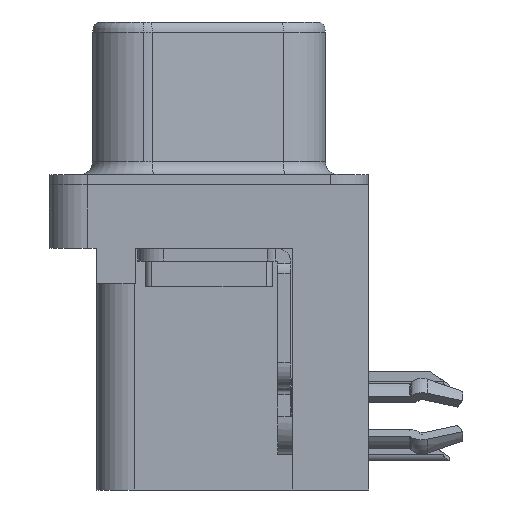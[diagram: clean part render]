
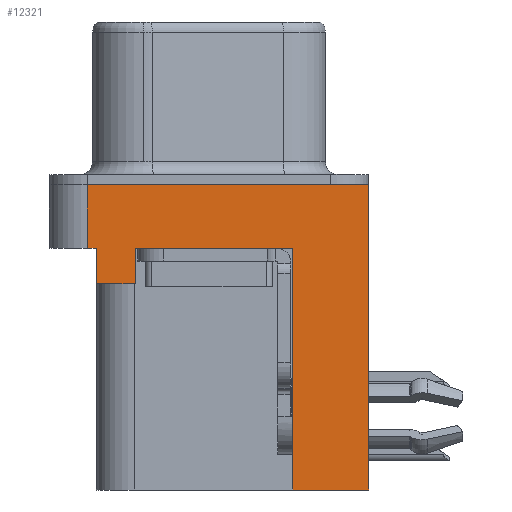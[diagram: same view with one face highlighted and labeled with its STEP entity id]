
A CAD part, left-side view. The second image highlights one B-rep face of the part: STEP entity #12321.
In plain terms, the highlighted planar face has unit normal (-1, 0, 0).
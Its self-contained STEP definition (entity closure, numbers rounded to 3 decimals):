
#18 = ORIENTED_EDGE ( 'NONE', *, *, #7341, .T. ) ;
#335 = CARTESIAN_POINT ( 'NONE',  ( -2.935, 4.775, -2.5 ) ) ;
#513 = CARTESIAN_POINT ( 'NONE',  ( -2.935, -3.295, -12. ) ) ;
#672 = VERTEX_POINT ( 'NONE', #10920 ) ;
#722 = DIRECTION ( 'NONE',  ( 0., 0., 1. ) ) ;
#1163 = CARTESIAN_POINT ( 'NONE',  ( -2.935, 2.895, -3.9 ) ) ;
#1334 = CARTESIAN_POINT ( 'NONE',  ( -2.935, -6.275, -2.5 ) ) ;
#1513 = ORIENTED_EDGE ( 'NONE', *, *, #6438, .F. ) ;
#1827 = VERTEX_POINT ( 'NONE', #1865 ) ;
#1865 = CARTESIAN_POINT ( 'NONE',  ( -2.935, 4.425, -3.9 ) ) ;
#2454 = AXIS2_PLACEMENT_3D ( 'NONE', #10579, #3220, #3462 ) ;
#2674 = LINE ( 'NONE', #13492, #13700 ) ;
#2811 = VECTOR ( 'NONE', #12744, 1000. ) ;
#2860 = LINE ( 'NONE', #6328, #15958 ) ;
#3008 = EDGE_CURVE ( 'NONE', #16433, #11795, #17096, .T. ) ;
#3125 = LINE ( 'NONE', #8642, #9172 ) ;
#3220 = DIRECTION ( 'NONE',  ( -1., 0., 0. ) ) ;
#3462 = DIRECTION ( 'NONE',  ( 0., 0., 1. ) ) ;
#3637 = CARTESIAN_POINT ( 'NONE',  ( -2.935, 2.895, -3.9 ) ) ;
#3792 = CARTESIAN_POINT ( 'NONE',  ( -2.935, 4.425, -3.9 ) ) ;
#3896 = CARTESIAN_POINT ( 'NONE',  ( -2.935, -6.275, -12. ) ) ;
#4034 = CARTESIAN_POINT ( 'NONE',  ( -2.935, -3.295, -12. ) ) ;
#4116 = LINE ( 'NONE', #3792, #15148 ) ;
#4424 = EDGE_CURVE ( 'NONE', #16189, #7552, #14632, .T. ) ;
#4591 = LINE ( 'NONE', #1334, #2811 ) ;
#5138 = VECTOR ( 'NONE', #6899, 1000. ) ;
#5188 = EDGE_CURVE ( 'NONE', #7552, #11795, #16511, .T. ) ;
#5221 = VECTOR ( 'NONE', #9967, 1000. ) ;
#5571 = VERTEX_POINT ( 'NONE', #3896 ) ;
#5678 = ORIENTED_EDGE ( 'NONE', *, *, #18589, .F. ) ;
#5716 = VERTEX_POINT ( 'NONE', #335 ) ;
#6162 = FACE_OUTER_BOUND ( 'NONE', #16030, .T. ) ;
#6328 = CARTESIAN_POINT ( 'NONE',  ( -2.935, -6.275, -2.5 ) ) ;
#6438 = EDGE_CURVE ( 'NONE', #1827, #12962, #2674, .T. ) ;
#6899 = DIRECTION ( 'NONE',  ( 0., 0., 1. ) ) ;
#7181 = CARTESIAN_POINT ( 'NONE',  ( -2.935, 4.775, -2.5 ) ) ;
#7341 = EDGE_CURVE ( 'NONE', #5716, #12962, #2860, .T. ) ;
#7552 = VERTEX_POINT ( 'NONE', #15807 ) ;
#7941 = CARTESIAN_POINT ( 'NONE',  ( -2.935, -3.295, -2.5 ) ) ;
#8073 = DIRECTION ( 'NONE',  ( 0., -1., 0. ) ) ;
#8179 = VERTEX_POINT ( 'NONE', #17858 ) ;
#8319 = VECTOR ( 'NONE', #17283, 1000. ) ;
#8461 = ORIENTED_EDGE ( 'NONE', *, *, #17868, .F. ) ;
#8642 = CARTESIAN_POINT ( 'NONE',  ( -2.935, -6.275, 0. ) ) ;
#8718 = EDGE_CURVE ( 'NONE', #5571, #672, #4591, .T. ) ;
#9172 = VECTOR ( 'NONE', #15888, 1000. ) ;
#9367 = VECTOR ( 'NONE', #18706, 1000. ) ;
#9967 = DIRECTION ( 'NONE',  ( 0., 0., 1. ) ) ;
#10202 = EDGE_CURVE ( 'NONE', #5716, #8179, #12670, .T. ) ;
#10428 = ORIENTED_EDGE ( 'NONE', *, *, #10202, .F. ) ;
#10579 = CARTESIAN_POINT ( 'NONE',  ( -2.935, -6.275, -2.5 ) ) ;
#10849 = DIRECTION ( 'NONE',  ( 0., 1., 0. ) ) ;
#10920 = CARTESIAN_POINT ( 'NONE',  ( -2.935, -6.275, 0. ) ) ;
#11165 = DIRECTION ( 'NONE',  ( 0., 1., 0. ) ) ;
#11351 = ORIENTED_EDGE ( 'NONE', *, *, #5188, .T. ) ;
#11795 = VERTEX_POINT ( 'NONE', #7941 ) ;
#12321 = ADVANCED_FACE ( 'NONE', ( #6162 ), #14818, .T. ) ;
#12621 = CARTESIAN_POINT ( 'NONE',  ( -2.935, 4.425, -2.5 ) ) ;
#12670 = LINE ( 'NONE', #7181, #5221 ) ;
#12744 = DIRECTION ( 'NONE',  ( 0., 0., 1. ) ) ;
#12962 = VERTEX_POINT ( 'NONE', #12621 ) ;
#13492 = CARTESIAN_POINT ( 'NONE',  ( -2.935, 4.425, -3.9 ) ) ;
#13700 = VECTOR ( 'NONE', #722, 1000. ) ;
#13840 = ORIENTED_EDGE ( 'NONE', *, *, #3008, .F. ) ;
#13915 = ORIENTED_EDGE ( 'NONE', *, *, #15385, .F. ) ;
#14632 = LINE ( 'NONE', #1163, #5138 ) ;
#14818 = PLANE ( 'NONE',  #2454 ) ;
#15148 = VECTOR ( 'NONE', #10849, 1000. ) ;
#15341 = ORIENTED_EDGE ( 'NONE', *, *, #8718, .T. ) ;
#15385 = EDGE_CURVE ( 'NONE', #5571, #16433, #17167, .T. ) ;
#15807 = CARTESIAN_POINT ( 'NONE',  ( -2.935, 2.895, -2.5 ) ) ;
#15826 = ORIENTED_EDGE ( 'NONE', *, *, #4424, .T. ) ;
#15888 = DIRECTION ( 'NONE',  ( 0., -1., 0. ) ) ;
#15958 = VECTOR ( 'NONE', #8073, 1000. ) ;
#16030 = EDGE_LOOP ( 'NONE', ( #5678, #10428, #18, #1513, #8461, #15826, #11351, #13840, #13915, #15341 ) ) ;
#16189 = VERTEX_POINT ( 'NONE', #3637 ) ;
#16433 = VERTEX_POINT ( 'NONE', #513 ) ;
#16511 = LINE ( 'NONE', #18621, #8319 ) ;
#16926 = CARTESIAN_POINT ( 'NONE',  ( -2.935, -3.295, -12. ) ) ;
#17096 = LINE ( 'NONE', #4034, #9367 ) ;
#17167 = LINE ( 'NONE', #16926, #18076 ) ;
#17283 = DIRECTION ( 'NONE',  ( 0., -1., 0. ) ) ;
#17858 = CARTESIAN_POINT ( 'NONE',  ( -2.935, 4.775, 0. ) ) ;
#17868 = EDGE_CURVE ( 'NONE', #16189, #1827, #4116, .T. ) ;
#18076 = VECTOR ( 'NONE', #11165, 1000. ) ;
#18589 = EDGE_CURVE ( 'NONE', #8179, #672, #3125, .T. ) ;
#18621 = CARTESIAN_POINT ( 'NONE',  ( -2.935, -6.275, -2.5 ) ) ;
#18706 = DIRECTION ( 'NONE',  ( 0., 0., 1. ) ) ;
